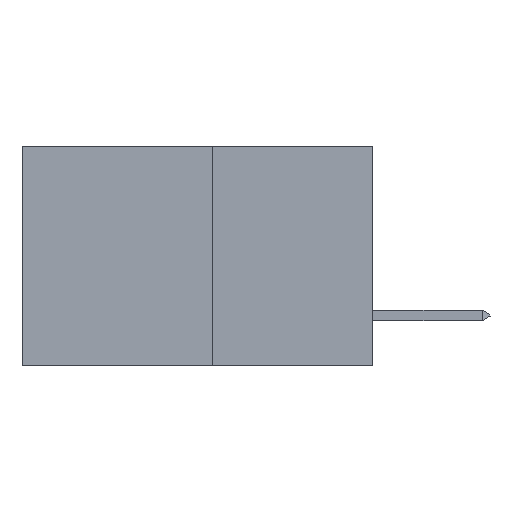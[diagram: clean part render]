
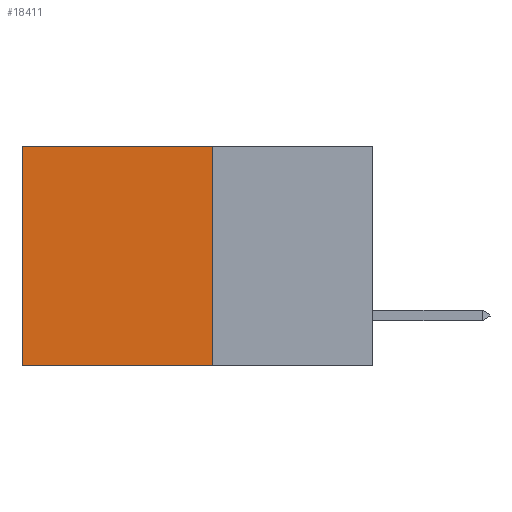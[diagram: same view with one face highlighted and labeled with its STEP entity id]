
A CAD part, left-side view. The second image highlights one B-rep face of the part: STEP entity #18411.
In plain terms, the highlighted planar face has unit normal (-1, 0, 0).
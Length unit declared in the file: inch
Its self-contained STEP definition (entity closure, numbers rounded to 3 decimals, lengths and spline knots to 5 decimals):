
#1092 = VERTEX_POINT ( 'NONE', #20139 ) ;
#1161 = EDGE_LOOP ( 'NONE', ( #30439, #13936, #33265, #10554 ) ) ;
#2954 = DIRECTION ( 'NONE',  ( 0., 0., -1. ) ) ;
#3131 = DIRECTION ( 'NONE',  ( 0., 0., -1. ) ) ;
#5446 = CARTESIAN_POINT ( 'NONE',  ( 0.277, 0.27, -0.37 ) ) ;
#5620 = DIRECTION ( 'NONE',  ( 0., 1., 0. ) ) ;
#6014 = CARTESIAN_POINT ( 'NONE',  ( 0.277, 0.59, -0.37 ) ) ;
#6653 = CARTESIAN_POINT ( 'NONE',  ( 0.277, 0.27, -0.37 ) ) ;
#10554 = ORIENTED_EDGE ( 'NONE', *, *, #27647, .T. ) ;
#10603 = PLANE ( 'NONE',  #23448 ) ;
#12539 = VECTOR ( 'NONE', #13707, 39.37008 ) ;
#12756 = CARTESIAN_POINT ( 'NONE',  ( 0.277, 0.27, -0.37 ) ) ;
#13707 = DIRECTION ( 'NONE',  ( 0., 0., -1. ) ) ;
#13936 = ORIENTED_EDGE ( 'NONE', *, *, #22721, .F. ) ;
#15795 = LINE ( 'NONE', #15925, #21885 ) ;
#15925 = CARTESIAN_POINT ( 'NONE',  ( 0.277, 0.27, -0.37 ) ) ;
#16513 = VECTOR ( 'NONE', #22072, 39.37008 ) ;
#18059 = CARTESIAN_POINT ( 'NONE',  ( 0.277, 0.59, 0. ) ) ;
#18375 = DIRECTION ( 'NONE',  ( 1., 0., 0. ) ) ;
#18411 = ADVANCED_FACE ( 'NONE', ( #23613 ), #10603, .F. ) ;
#19446 = LINE ( 'NONE', #6014, #12539 ) ;
#20139 = CARTESIAN_POINT ( 'NONE',  ( 0.277, 0.59, -0.37 ) ) ;
#21630 = LINE ( 'NONE', #31294, #27670 ) ;
#21885 = VECTOR ( 'NONE', #3131, 39.37008 ) ;
#21970 = EDGE_CURVE ( 'NONE', #25808, #1092, #19446, .T. ) ;
#22072 = DIRECTION ( 'NONE',  ( 0., 1., 0. ) ) ;
#22721 = EDGE_CURVE ( 'NONE', #32886, #1092, #29460, .T. ) ;
#22760 = CARTESIAN_POINT ( 'NONE',  ( 0.277, 0.27, 0. ) ) ;
#23448 = AXIS2_PLACEMENT_3D ( 'NONE', #5446, #18375, #2954 ) ;
#23613 = FACE_OUTER_BOUND ( 'NONE', #1161, .T. ) ;
#25808 = VERTEX_POINT ( 'NONE', #18059 ) ;
#27647 = EDGE_CURVE ( 'NONE', #31591, #25808, #21630, .T. ) ;
#27670 = VECTOR ( 'NONE', #5620, 39.37008 ) ;
#29460 = LINE ( 'NONE', #6653, #16513 ) ;
#29542 = EDGE_CURVE ( 'NONE', #31591, #32886, #15795, .T. ) ;
#30439 = ORIENTED_EDGE ( 'NONE', *, *, #21970, .T. ) ;
#31294 = CARTESIAN_POINT ( 'NONE',  ( 0.277, 0.27, 0. ) ) ;
#31591 = VERTEX_POINT ( 'NONE', #22760 ) ;
#32886 = VERTEX_POINT ( 'NONE', #12756 ) ;
#33265 = ORIENTED_EDGE ( 'NONE', *, *, #29542, .F. ) ;
